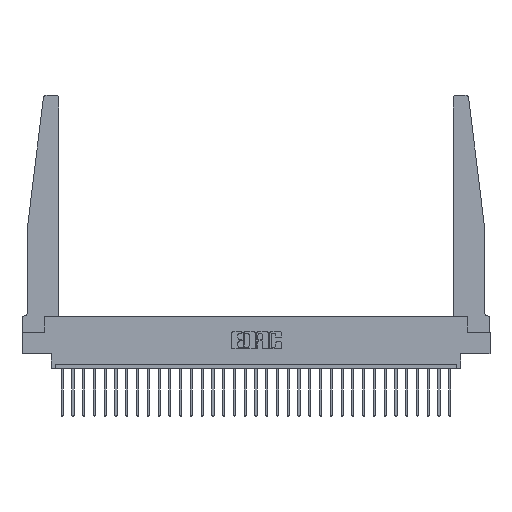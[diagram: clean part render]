
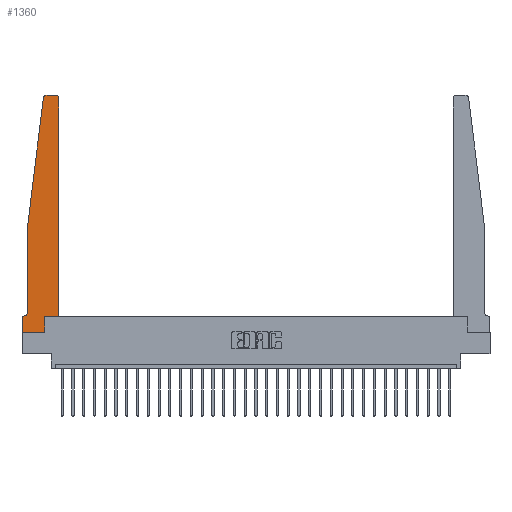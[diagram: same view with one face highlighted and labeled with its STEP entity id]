
A CAD part, top view. The second image highlights one B-rep face of the part: STEP entity #1360.
In plain terms, the highlighted planar face has unit normal (0, 0, 1).
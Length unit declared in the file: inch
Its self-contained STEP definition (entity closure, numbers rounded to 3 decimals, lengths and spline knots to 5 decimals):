
#144 = CIRCLE ( 'NONE', #10642, 0.03 ) ;
#648 = EDGE_CURVE ( 'NONE', #9973, #20133, #17235, .T. ) ;
#1248 = ORIENTED_EDGE ( 'NONE', *, *, #6267, .T. ) ;
#1360 = ADVANCED_FACE ( 'NONE', ( #5856 ), #3856, .T. ) ;
#2832 = EDGE_CURVE ( 'NONE', #19866, #21461, #21891, .T. ) ;
#3270 = VERTEX_POINT ( 'NONE', #22187 ) ;
#3354 = AXIS2_PLACEMENT_3D ( 'NONE', #17097, #17279, #4322 ) ;
#3537 = EDGE_CURVE ( 'NONE', #10882, #3270, #17076, .T. ) ;
#3856 = PLANE ( 'NONE',  #5795 ) ;
#4045 = CARTESIAN_POINT ( 'NONE',  ( 0.27653, 2.72, 0.37 ) ) ;
#4166 = CARTESIAN_POINT ( 'NONE',  ( 0.2605, 0.18, 0.37 ) ) ;
#4169 = VECTOR ( 'NONE', #7790, 39.37008 ) ;
#4322 = DIRECTION ( 'NONE',  ( -1., 0., 0. ) ) ;
#4465 = DIRECTION ( 'NONE',  ( 0., 1., 0. ) ) ;
#4514 = DIRECTION ( 'NONE',  ( -1., 0., 0. ) ) ;
#4564 = AXIS2_PLACEMENT_3D ( 'NONE', #4045, #8582, #8477 ) ;
#4753 = VERTEX_POINT ( 'NONE', #7958 ) ;
#4823 = CARTESIAN_POINT ( 'NONE',  ( 0., 0.1875, 0.37 ) ) ;
#5328 = LINE ( 'NONE', #11649, #20088 ) ;
#5605 = VERTEX_POINT ( 'NONE', #13318 ) ;
#5630 = CARTESIAN_POINT ( 'NONE',  ( 0.065, 1.25, 0.37 ) ) ;
#5795 = AXIS2_PLACEMENT_3D ( 'NONE', #21150, #27844, #21257 ) ;
#5856 = FACE_OUTER_BOUND ( 'NONE', #8776, .T. ) ;
#6155 = DIRECTION ( 'NONE',  ( 0., 0., 1. ) ) ;
#6183 = EDGE_CURVE ( 'NONE', #24427, #9817, #25671, .T. ) ;
#6267 = EDGE_CURVE ( 'NONE', #17801, #5605, #9153, .T. ) ;
#6605 = CARTESIAN_POINT ( 'NONE',  ( 0.2605, 0., 0.37 ) ) ;
#6729 = DIRECTION ( 'NONE',  ( 0., -1., 0. ) ) ;
#6735 = VECTOR ( 'NONE', #6729, 39.37008 ) ;
#6816 = DIRECTION ( 'NONE',  ( 1., 0., 0. ) ) ;
#6966 = LINE ( 'NONE', #17666, #23116 ) ;
#7045 = CARTESIAN_POINT ( 'NONE',  ( 0.27653, 2.75, 0.37 ) ) ;
#7120 = ORIENTED_EDGE ( 'NONE', *, *, #2832, .T. ) ;
#7304 = ORIENTED_EDGE ( 'NONE', *, *, #13199, .T. ) ;
#7790 = DIRECTION ( 'NONE',  ( -1., 0., 0. ) ) ;
#7958 = CARTESIAN_POINT ( 'NONE',  ( 0.015, 0.1875, 0.37 ) ) ;
#8477 = DIRECTION ( 'NONE',  ( 1., 0., 0. ) ) ;
#8582 = DIRECTION ( 'NONE',  ( 0., 0., 1. ) ) ;
#8776 = EDGE_LOOP ( 'NONE', ( #14126, #28463, #28150, #7120, #13685, #13163, #28405, #7304, #1248, #14738, #22493, #25154 ) ) ;
#8944 = CARTESIAN_POINT ( 'NONE',  ( 0., 0., 0.37 ) ) ;
#8977 = EDGE_CURVE ( 'NONE', #21461, #4753, #15866, .T. ) ;
#9010 = VECTOR ( 'NONE', #6816, 39.37008 ) ;
#9153 = LINE ( 'NONE', #4166, #18063 ) ;
#9817 = VERTEX_POINT ( 'NONE', #9827 ) ;
#9827 = CARTESIAN_POINT ( 'NONE',  ( 0., 0., 0.37 ) ) ;
#9973 = VERTEX_POINT ( 'NONE', #25505 ) ;
#10642 = AXIS2_PLACEMENT_3D ( 'NONE', #19573, #6155, #12866 ) ;
#10882 = VERTEX_POINT ( 'NONE', #12871 ) ;
#11335 = CARTESIAN_POINT ( 'NONE',  ( 0.425, 0.18, 0.37 ) ) ;
#11503 = CARTESIAN_POINT ( 'NONE',  ( 0.065, 0.2375, 0.37 ) ) ;
#11649 = CARTESIAN_POINT ( 'NONE',  ( 0.065, 1.25, 0.37 ) ) ;
#11766 = CARTESIAN_POINT ( 'NONE',  ( 0.065, 1.25, 0.37 ) ) ;
#12080 = LINE ( 'NONE', #11335, #9010 ) ;
#12277 = LINE ( 'NONE', #8944, #14361 ) ;
#12866 = DIRECTION ( 'NONE',  ( 1., 0., 0. ) ) ;
#12871 = CARTESIAN_POINT ( 'NONE',  ( 0.425, 0.18, 0.37 ) ) ;
#13163 = ORIENTED_EDGE ( 'NONE', *, *, #16125, .T. ) ;
#13199 = EDGE_CURVE ( 'NONE', #9817, #17801, #12277, .T. ) ;
#13318 = CARTESIAN_POINT ( 'NONE',  ( 0.2605, 0.18, 0.37 ) ) ;
#13685 = ORIENTED_EDGE ( 'NONE', *, *, #8977, .T. ) ;
#14126 = ORIENTED_EDGE ( 'NONE', *, *, #648, .T. ) ;
#14361 = VECTOR ( 'NONE', #15816, 39.37008 ) ;
#14590 = EDGE_CURVE ( 'NONE', #19388, #19866, #5328, .T. ) ;
#14738 = ORIENTED_EDGE ( 'NONE', *, *, #16991, .T. ) ;
#15365 = VECTOR ( 'NONE', #21013, 39.37008 ) ;
#15816 = DIRECTION ( 'NONE',  ( 1., 0., 0. ) ) ;
#15866 = CIRCLE ( 'NONE', #3354, 0.05 ) ;
#16125 = EDGE_CURVE ( 'NONE', #4753, #24427, #6966, .T. ) ;
#16991 = EDGE_CURVE ( 'NONE', #5605, #10882, #12080, .T. ) ;
#17076 = LINE ( 'NONE', #18528, #18137 ) ;
#17097 = CARTESIAN_POINT ( 'NONE',  ( 0.015, 0.2375, 0.37 ) ) ;
#17235 = LINE ( 'NONE', #27999, #4169 ) ;
#17279 = DIRECTION ( 'NONE',  ( 0., 0., -1. ) ) ;
#17666 = CARTESIAN_POINT ( 'NONE',  ( 0.065, 0.1875, 0.37 ) ) ;
#17801 = VERTEX_POINT ( 'NONE', #6605 ) ;
#18063 = VECTOR ( 'NONE', #4465, 39.37008 ) ;
#18137 = VECTOR ( 'NONE', #22836, 39.37008 ) ;
#18261 = DIRECTION ( 'NONE',  ( -0.122, -0.992, 0. ) ) ;
#18528 = CARTESIAN_POINT ( 'NONE',  ( 0.425, 0.18, 0.37 ) ) ;
#19388 = VERTEX_POINT ( 'NONE', #20054 ) ;
#19573 = CARTESIAN_POINT ( 'NONE',  ( 0.395, 2.72, 0.37 ) ) ;
#19866 = VERTEX_POINT ( 'NONE', #11766 ) ;
#20054 = CARTESIAN_POINT ( 'NONE',  ( 0.24675, 2.72367, 0.37 ) ) ;
#20088 = VECTOR ( 'NONE', #18261, 39.37008 ) ;
#20133 = VERTEX_POINT ( 'NONE', #7045 ) ;
#21013 = DIRECTION ( 'NONE',  ( 0., -1., 0. ) ) ;
#21150 = CARTESIAN_POINT ( 'NONE',  ( 0., 0.1875, 0.37 ) ) ;
#21257 = DIRECTION ( 'NONE',  ( 1., 0., 0. ) ) ;
#21461 = VERTEX_POINT ( 'NONE', #11503 ) ;
#21891 = LINE ( 'NONE', #5630, #15365 ) ;
#22187 = CARTESIAN_POINT ( 'NONE',  ( 0.425, 2.72, 0.37 ) ) ;
#22493 = ORIENTED_EDGE ( 'NONE', *, *, #3537, .T. ) ;
#22836 = DIRECTION ( 'NONE',  ( 0., 1., 0. ) ) ;
#23116 = VECTOR ( 'NONE', #4514, 39.37008 ) ;
#23866 = CIRCLE ( 'NONE', #4564, 0.03 ) ;
#24427 = VERTEX_POINT ( 'NONE', #4823 ) ;
#25154 = ORIENTED_EDGE ( 'NONE', *, *, #26564, .T. ) ;
#25505 = CARTESIAN_POINT ( 'NONE',  ( 0.395, 2.75, 0.37 ) ) ;
#25671 = LINE ( 'NONE', #26736, #6735 ) ;
#26564 = EDGE_CURVE ( 'NONE', #3270, #9973, #144, .T. ) ;
#26736 = CARTESIAN_POINT ( 'NONE',  ( 0., 0., 0.37 ) ) ;
#27104 = EDGE_CURVE ( 'NONE', #20133, #19388, #23866, .T. ) ;
#27844 = DIRECTION ( 'NONE',  ( 0., 0., 1. ) ) ;
#27999 = CARTESIAN_POINT ( 'NONE',  ( 0.25, 2.75, 0.37 ) ) ;
#28150 = ORIENTED_EDGE ( 'NONE', *, *, #14590, .T. ) ;
#28405 = ORIENTED_EDGE ( 'NONE', *, *, #6183, .T. ) ;
#28463 = ORIENTED_EDGE ( 'NONE', *, *, #27104, .T. ) ;
